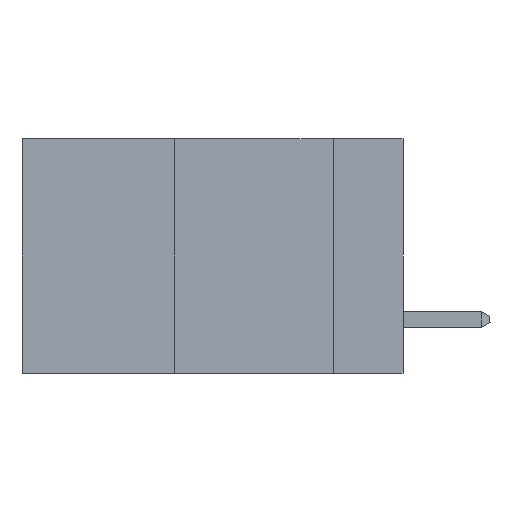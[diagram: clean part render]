
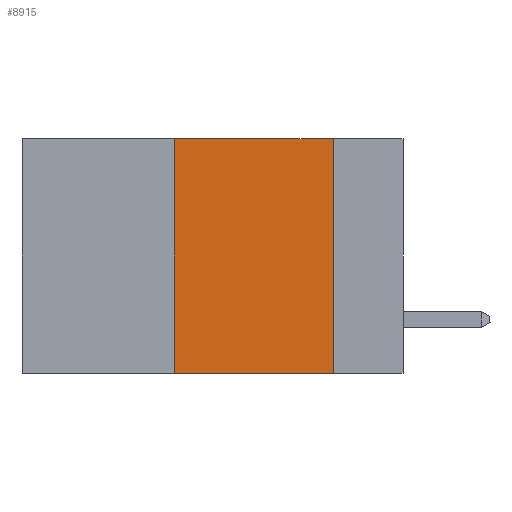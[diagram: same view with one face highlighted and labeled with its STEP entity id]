
A CAD part, left-side view. The second image highlights one B-rep face of the part: STEP entity #8915.
In plain terms, the highlighted planar face has unit normal (-1, 0, 0).
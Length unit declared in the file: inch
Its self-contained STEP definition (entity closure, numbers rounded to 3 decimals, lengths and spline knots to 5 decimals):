
#46 = VECTOR ( 'NONE', #649, 39.37008 ) ;
#442 = VERTEX_POINT ( 'NONE', #4606 ) ;
#611 = CARTESIAN_POINT ( 'NONE',  ( 0., 0.6, -0.37 ) ) ;
#642 = DIRECTION ( 'NONE',  ( 0., -1., 0. ) ) ;
#649 = DIRECTION ( 'NONE',  ( 0., -1., 0. ) ) ;
#1385 = VERTEX_POINT ( 'NONE', #5450 ) ;
#2074 = ORIENTED_EDGE ( 'NONE', *, *, #8164, .F. ) ;
#2106 = VECTOR ( 'NONE', #2428, 39.37008 ) ;
#2285 = LINE ( 'NONE', #8587, #6802 ) ;
#2428 = DIRECTION ( 'NONE',  ( 0., 0., 1. ) ) ;
#2629 = EDGE_CURVE ( 'NONE', #8694, #1385, #2650, .T. ) ;
#2650 = LINE ( 'NONE', #611, #46 ) ;
#3146 = DIRECTION ( 'NONE',  ( 0., 0., -1. ) ) ;
#3217 = AXIS2_PLACEMENT_3D ( 'NONE', #6592, #7524, #3146 ) ;
#3332 = DIRECTION ( 'NONE',  ( 0., 0., -1. ) ) ;
#3888 = LINE ( 'NONE', #7759, #9261 ) ;
#4606 = CARTESIAN_POINT ( 'NONE',  ( 0., 0.36, 0. ) ) ;
#4965 = ORIENTED_EDGE ( 'NONE', *, *, #2629, .T. ) ;
#5450 = CARTESIAN_POINT ( 'NONE',  ( 0., 0.11, -0.37 ) ) ;
#5633 = EDGE_CURVE ( 'NONE', #442, #6827, #2285, .T. ) ;
#6592 = CARTESIAN_POINT ( 'NONE',  ( 0., 0.6, 0. ) ) ;
#6617 = LINE ( 'NONE', #10335, #2106 ) ;
#6802 = VECTOR ( 'NONE', #642, 39.37008 ) ;
#6827 = VERTEX_POINT ( 'NONE', #9317 ) ;
#7524 = DIRECTION ( 'NONE',  ( 1., 0., 0. ) ) ;
#7590 = ORIENTED_EDGE ( 'NONE', *, *, #5633, .F. ) ;
#7759 = CARTESIAN_POINT ( 'NONE',  ( 0., 0.11, 0. ) ) ;
#7987 = EDGE_CURVE ( 'NONE', #8694, #442, #6617, .T. ) ;
#8164 = EDGE_CURVE ( 'NONE', #6827, #1385, #3888, .T. ) ;
#8587 = CARTESIAN_POINT ( 'NONE',  ( 0., 0.6, 0. ) ) ;
#8694 = VERTEX_POINT ( 'NONE', #9345 ) ;
#8712 = ORIENTED_EDGE ( 'NONE', *, *, #7987, .F. ) ;
#8915 = ADVANCED_FACE ( 'NONE', ( #9236 ), #9384, .F. ) ;
#9236 = FACE_OUTER_BOUND ( 'NONE', #10111, .T. ) ;
#9261 = VECTOR ( 'NONE', #3332, 39.37008 ) ;
#9317 = CARTESIAN_POINT ( 'NONE',  ( 0., 0.11, 0. ) ) ;
#9345 = CARTESIAN_POINT ( 'NONE',  ( 0., 0.36, -0.37 ) ) ;
#9384 = PLANE ( 'NONE',  #3217 ) ;
#10111 = EDGE_LOOP ( 'NONE', ( #2074, #7590, #8712, #4965 ) ) ;
#10335 = CARTESIAN_POINT ( 'NONE',  ( 0., 0.36, 0. ) ) ;
